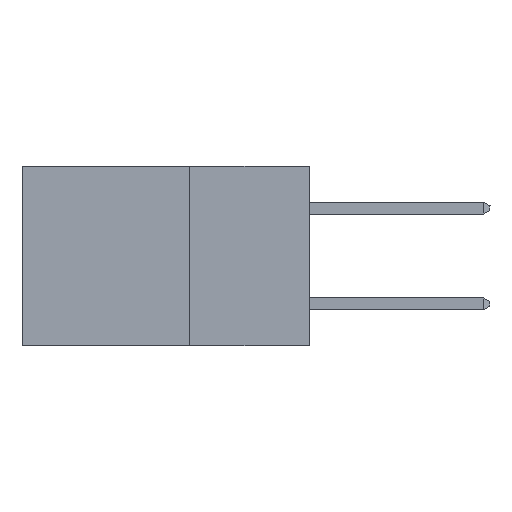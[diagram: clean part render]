
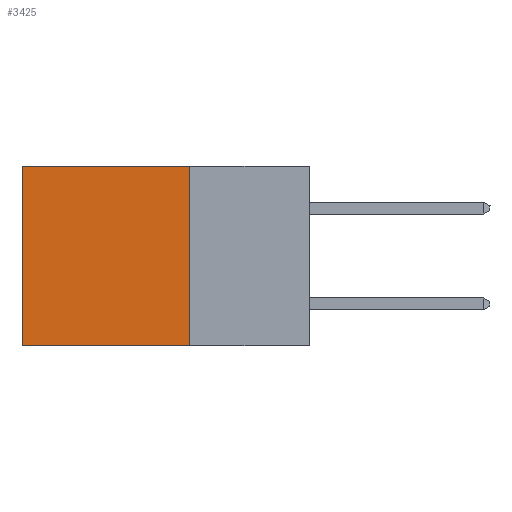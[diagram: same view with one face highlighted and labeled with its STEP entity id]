
A CAD part, left-side view. The second image highlights one B-rep face of the part: STEP entity #3425.
In plain terms, the highlighted planar face has unit normal (-1, 0, 0).
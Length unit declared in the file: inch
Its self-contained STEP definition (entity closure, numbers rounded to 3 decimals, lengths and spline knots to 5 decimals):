
#153 = CARTESIAN_POINT ( 'NONE',  ( 0.2875, 0.25, -0.375 ) ) ;
#364 = CARTESIAN_POINT ( 'NONE',  ( 0.2875, 0.6, 0. ) ) ;
#459 = EDGE_CURVE ( 'NONE', #12494, #12720, #4124, .T. ) ;
#735 = DIRECTION ( 'NONE',  ( 1., 0., 0. ) ) ;
#868 = CARTESIAN_POINT ( 'NONE',  ( 0.2875, 0.25, -0.375 ) ) ;
#1099 = ORIENTED_EDGE ( 'NONE', *, *, #9615, .T. ) ;
#1439 = CARTESIAN_POINT ( 'NONE',  ( 0.2875, 0.6, -0.375 ) ) ;
#1954 = ORIENTED_EDGE ( 'NONE', *, *, #9746, .F. ) ;
#2580 = DIRECTION ( 'NONE',  ( 0., 0., -1. ) ) ;
#2798 = DIRECTION ( 'NONE',  ( 0., 1., 0. ) ) ;
#3425 = ADVANCED_FACE ( 'NONE', ( #12404 ), #14823, .F. ) ;
#3629 = CARTESIAN_POINT ( 'NONE',  ( 0.2875, 0.25, -0.375 ) ) ;
#3694 = CARTESIAN_POINT ( 'NONE',  ( 0.2875, 0.6, -0.375 ) ) ;
#4124 = LINE ( 'NONE', #12197, #9291 ) ;
#5451 = VECTOR ( 'NONE', #2580, 39.37008 ) ;
#5669 = LINE ( 'NONE', #8927, #9360 ) ;
#5906 = VERTEX_POINT ( 'NONE', #153 ) ;
#6563 = EDGE_LOOP ( 'NONE', ( #1099, #1954, #9593, #8641 ) ) ;
#6636 = CARTESIAN_POINT ( 'NONE',  ( 0.2875, 0.25, 0. ) ) ;
#7599 = DIRECTION ( 'NONE',  ( 0., 1., 0. ) ) ;
#7914 = AXIS2_PLACEMENT_3D ( 'NONE', #868, #735, #12338 ) ;
#8641 = ORIENTED_EDGE ( 'NONE', *, *, #459, .T. ) ;
#8927 = CARTESIAN_POINT ( 'NONE',  ( 0.2875, 0.25, -0.375 ) ) ;
#9291 = VECTOR ( 'NONE', #7599, 39.37008 ) ;
#9360 = VECTOR ( 'NONE', #10276, 39.37008 ) ;
#9593 = ORIENTED_EDGE ( 'NONE', *, *, #13333, .F. ) ;
#9615 = EDGE_CURVE ( 'NONE', #12720, #11369, #12836, .T. ) ;
#9746 = EDGE_CURVE ( 'NONE', #5906, #11369, #13981, .T. ) ;
#10276 = DIRECTION ( 'NONE',  ( 0., 0., -1. ) ) ;
#11369 = VERTEX_POINT ( 'NONE', #1439 ) ;
#12197 = CARTESIAN_POINT ( 'NONE',  ( 0.2875, 0.25, 0. ) ) ;
#12338 = DIRECTION ( 'NONE',  ( 0., 0., -1. ) ) ;
#12404 = FACE_OUTER_BOUND ( 'NONE', #6563, .T. ) ;
#12494 = VERTEX_POINT ( 'NONE', #6636 ) ;
#12720 = VERTEX_POINT ( 'NONE', #364 ) ;
#12836 = LINE ( 'NONE', #3694, #5451 ) ;
#13333 = EDGE_CURVE ( 'NONE', #12494, #5906, #5669, .T. ) ;
#13890 = VECTOR ( 'NONE', #2798, 39.37008 ) ;
#13981 = LINE ( 'NONE', #3629, #13890 ) ;
#14823 = PLANE ( 'NONE',  #7914 ) ;
